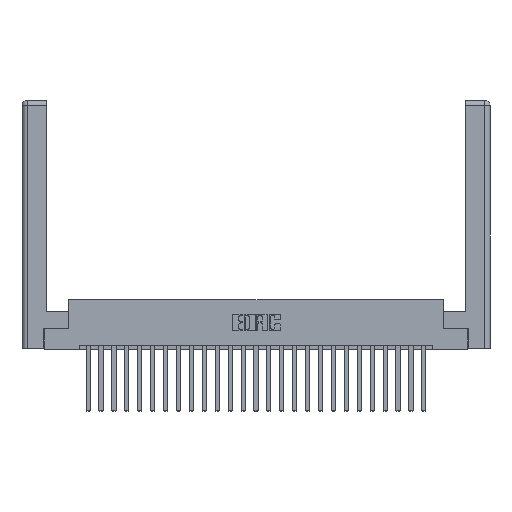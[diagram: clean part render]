
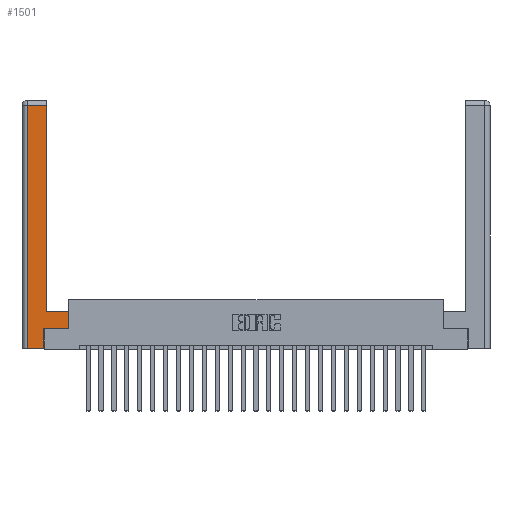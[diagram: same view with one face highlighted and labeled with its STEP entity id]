
A CAD part, top view. The second image highlights one B-rep face of the part: STEP entity #1501.
In plain terms, the highlighted planar face has unit normal (0, 0, 1).
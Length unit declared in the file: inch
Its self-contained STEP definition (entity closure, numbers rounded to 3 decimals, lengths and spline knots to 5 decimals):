
#191 = CARTESIAN_POINT ( 'NONE',  ( 0.295, 0.45, 0. ) ) ;
#638 = CARTESIAN_POINT ( 'NONE',  ( 0.295, 2.94, 0. ) ) ;
#807 = ORIENTED_EDGE ( 'NONE', *, *, #16273, .T. ) ;
#1501 = ADVANCED_FACE ( 'NONE', ( #24333 ), #13131, .F. ) ;
#1611 = ORIENTED_EDGE ( 'NONE', *, *, #17356, .T. ) ;
#2560 = DIRECTION ( 'NONE',  ( 0., -1., 0. ) ) ;
#3959 = ORIENTED_EDGE ( 'NONE', *, *, #18636, .T. ) ;
#4151 = VERTEX_POINT ( 'NONE', #12332 ) ;
#4274 = DIRECTION ( 'NONE',  ( 0., 1., 0. ) ) ;
#4415 = CARTESIAN_POINT ( 'NONE',  ( 0.265, 0.245, 0. ) ) ;
#5201 = VECTOR ( 'NONE', #2560, 39.37008 ) ;
#5209 = ORIENTED_EDGE ( 'NONE', *, *, #12126, .T. ) ;
#6212 = VERTEX_POINT ( 'NONE', #19130 ) ;
#6220 = DIRECTION ( 'NONE',  ( 1., 0., 0. ) ) ;
#6239 = ORIENTED_EDGE ( 'NONE', *, *, #21127, .T. ) ;
#7067 = CARTESIAN_POINT ( 'NONE',  ( 0., 0., 0. ) ) ;
#7344 = VECTOR ( 'NONE', #17317, 39.37008 ) ;
#7652 = CARTESIAN_POINT ( 'NONE',  ( 0.265, 0.245, 0. ) ) ;
#9095 = VERTEX_POINT ( 'NONE', #14633 ) ;
#9287 = LINE ( 'NONE', #20491, #14819 ) ;
#11343 = DIRECTION ( 'NONE',  ( -1., 0., 0. ) ) ;
#11592 = EDGE_CURVE ( 'NONE', #24223, #19282, #12233, .T. ) ;
#11786 = EDGE_CURVE ( 'NONE', #20487, #6212, #25061, .T. ) ;
#12038 = LINE ( 'NONE', #15800, #14190 ) ;
#12050 = CARTESIAN_POINT ( 'NONE',  ( 0.0615, 2.94, 0. ) ) ;
#12126 = EDGE_CURVE ( 'NONE', #4151, #9095, #19222, .T. ) ;
#12163 = VECTOR ( 'NONE', #18498, 39.37008 ) ;
#12233 = LINE ( 'NONE', #7652, #7344 ) ;
#12332 = CARTESIAN_POINT ( 'NONE',  ( 0.565, 0.45, 0. ) ) ;
#13131 = PLANE ( 'NONE',  #13137 ) ;
#13137 = AXIS2_PLACEMENT_3D ( 'NONE', #7067, #22990, #11343 ) ;
#13358 = CARTESIAN_POINT ( 'NONE',  ( 0.265, 0., 0. ) ) ;
#14190 = VECTOR ( 'NONE', #6220, 39.37008 ) ;
#14306 = CARTESIAN_POINT ( 'NONE',  ( 0.0615, 0., 0. ) ) ;
#14633 = CARTESIAN_POINT ( 'NONE',  ( 0.295, 0.45, 0. ) ) ;
#14819 = VECTOR ( 'NONE', #22542, 39.37008 ) ;
#14833 = CARTESIAN_POINT ( 'NONE',  ( 0.0615, 2.94, 0. ) ) ;
#15017 = DIRECTION ( 'NONE',  ( 0., 1., 0. ) ) ;
#15076 = CARTESIAN_POINT ( 'NONE',  ( 0.565, 0.245, 0. ) ) ;
#15800 = CARTESIAN_POINT ( 'NONE',  ( 0.565, 0.245, 0. ) ) ;
#15890 = DIRECTION ( 'NONE',  ( -1., 0., 0. ) ) ;
#16265 = ORIENTED_EDGE ( 'NONE', *, *, #11592, .T. ) ;
#16273 = EDGE_CURVE ( 'NONE', #24448, #20487, #19807, .T. ) ;
#16761 = ORIENTED_EDGE ( 'NONE', *, *, #11786, .T. ) ;
#17022 = LINE ( 'NONE', #19730, #23378 ) ;
#17281 = EDGE_LOOP ( 'NONE', ( #19606, #807, #16761, #3959, #16265, #6239, #1611, #5209 ) ) ;
#17317 = DIRECTION ( 'NONE',  ( 0., 1., 0. ) ) ;
#17356 = EDGE_CURVE ( 'NONE', #20218, #4151, #17022, .T. ) ;
#17496 = LINE ( 'NONE', #20777, #22342 ) ;
#18498 = DIRECTION ( 'NONE',  ( -1., 0., 0. ) ) ;
#18636 = EDGE_CURVE ( 'NONE', #6212, #24223, #9287, .T. ) ;
#19130 = CARTESIAN_POINT ( 'NONE',  ( 0.0615, 0., 0. ) ) ;
#19222 = LINE ( 'NONE', #191, #22876 ) ;
#19282 = VERTEX_POINT ( 'NONE', #4415 ) ;
#19606 = ORIENTED_EDGE ( 'NONE', *, *, #19623, .T. ) ;
#19623 = EDGE_CURVE ( 'NONE', #9095, #24448, #17496, .T. ) ;
#19730 = CARTESIAN_POINT ( 'NONE',  ( 0.565, 0.45, 0. ) ) ;
#19807 = LINE ( 'NONE', #14833, #12163 ) ;
#20218 = VERTEX_POINT ( 'NONE', #15076 ) ;
#20487 = VERTEX_POINT ( 'NONE', #12050 ) ;
#20491 = CARTESIAN_POINT ( 'NONE',  ( 0.265, 0., 0. ) ) ;
#20777 = CARTESIAN_POINT ( 'NONE',  ( 0.295, 3., 0. ) ) ;
#21127 = EDGE_CURVE ( 'NONE', #19282, #20218, #12038, .T. ) ;
#22342 = VECTOR ( 'NONE', #15017, 39.37008 ) ;
#22542 = DIRECTION ( 'NONE',  ( 1., 0., 0. ) ) ;
#22876 = VECTOR ( 'NONE', #15890, 39.37008 ) ;
#22990 = DIRECTION ( 'NONE',  ( 0., 0., -1. ) ) ;
#23378 = VECTOR ( 'NONE', #4274, 39.37008 ) ;
#24223 = VERTEX_POINT ( 'NONE', #13358 ) ;
#24333 = FACE_OUTER_BOUND ( 'NONE', #17281, .T. ) ;
#24448 = VERTEX_POINT ( 'NONE', #638 ) ;
#25061 = LINE ( 'NONE', #14306, #5201 ) ;
